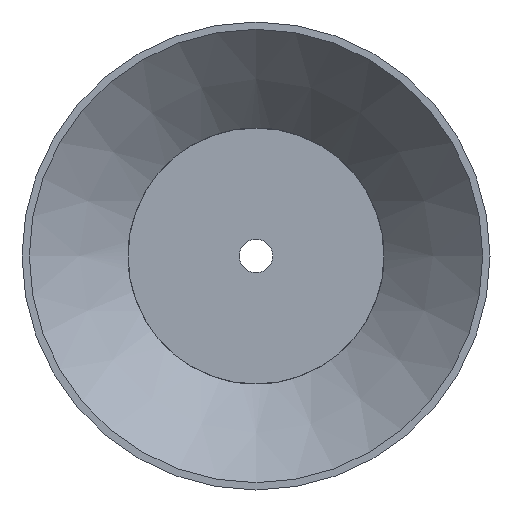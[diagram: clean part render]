
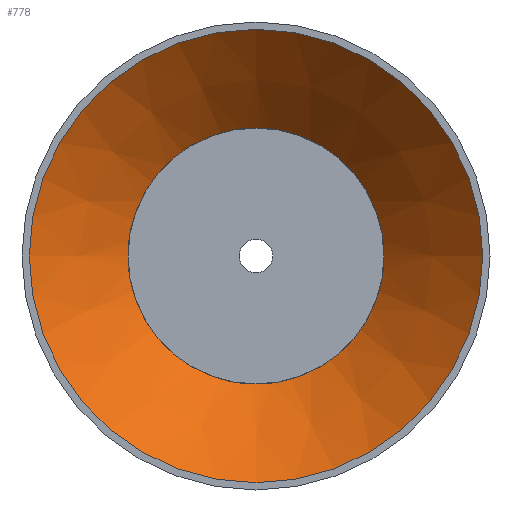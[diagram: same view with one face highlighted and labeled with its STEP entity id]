
A CAD part, front view. The second image highlights one B-rep face of the part: STEP entity #778.
In plain terms, the highlighted conical face has half-angle 44.201 degrees and reference radius 30.725 mm.
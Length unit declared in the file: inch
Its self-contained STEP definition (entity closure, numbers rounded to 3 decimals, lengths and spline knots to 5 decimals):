
#110=(
BOUNDED_CURVE()
B_SPLINE_CURVE(2,(#1062,#1063,#1064),.UNSPECIFIED.,.F.,.F.)
B_SPLINE_CURVE_WITH_KNOTS((3,3),(0.,0.02415),.UNSPECIFIED.)
CURVE()
GEOMETRIC_REPRESENTATION_ITEM()
RATIONAL_B_SPLINE_CURVE((1.,1.,1.))
REPRESENTATION_ITEM('')
);
#111=(
BOUNDED_CURVE()
B_SPLINE_CURVE(2,(#1066,#1067,#1068),.UNSPECIFIED.,.F.,.F.)
B_SPLINE_CURVE_WITH_KNOTS((3,3),(1.03572,1.05987),
 .UNSPECIFIED.)
CURVE()
GEOMETRIC_REPRESENTATION_ITEM()
RATIONAL_B_SPLINE_CURVE((1.,1.,1.))
REPRESENTATION_ITEM('')
);
#112=(
BOUNDED_CURVE()
B_SPLINE_CURVE(2,(#1071,#1072,#1073),.UNSPECIFIED.,.F.,.F.)
B_SPLINE_CURVE_WITH_KNOTS((3,3),(0.,0.02414),.UNSPECIFIED.)
CURVE()
GEOMETRIC_REPRESENTATION_ITEM()
RATIONAL_B_SPLINE_CURVE((1.,1.,1.))
REPRESENTATION_ITEM('')
);
#113=(
BOUNDED_CURVE()
B_SPLINE_CURVE(2,(#1075,#1076,#1077),.UNSPECIFIED.,.F.,.F.)
B_SPLINE_CURVE_WITH_KNOTS((3,3),(1.03572,1.05987),
 .UNSPECIFIED.)
CURVE()
GEOMETRIC_REPRESENTATION_ITEM()
RATIONAL_B_SPLINE_CURVE((1.,1.,1.))
REPRESENTATION_ITEM('')
);
#114=(
BOUNDED_CURVE()
B_SPLINE_CURVE(2,(#1080,#1081,#1082),.UNSPECIFIED.,.F.,.F.)
B_SPLINE_CURVE_WITH_KNOTS((3,3),(0.,0.02414),.UNSPECIFIED.)
CURVE()
GEOMETRIC_REPRESENTATION_ITEM()
RATIONAL_B_SPLINE_CURVE((1.,1.,1.))
REPRESENTATION_ITEM('')
);
#115=(
BOUNDED_CURVE()
B_SPLINE_CURVE(2,(#1084,#1085,#1086),.UNSPECIFIED.,.F.,.F.)
B_SPLINE_CURVE_WITH_KNOTS((3,3),(1.03578,1.05992),
 .UNSPECIFIED.)
CURVE()
GEOMETRIC_REPRESENTATION_ITEM()
RATIONAL_B_SPLINE_CURVE((1.,1.,1.))
REPRESENTATION_ITEM('')
);
#116=(
BOUNDED_CURVE()
B_SPLINE_CURVE(2,(#1090,#1091,#1092),.UNSPECIFIED.,.F.,.F.)
B_SPLINE_CURVE_WITH_KNOTS((3,3),(0.,0.02414),.UNSPECIFIED.)
CURVE()
GEOMETRIC_REPRESENTATION_ITEM()
RATIONAL_B_SPLINE_CURVE((1.,1.,1.))
REPRESENTATION_ITEM('')
);
#117=(
BOUNDED_CURVE()
B_SPLINE_CURVE(2,(#1096,#1097,#1098),.UNSPECIFIED.,.F.,.F.)
B_SPLINE_CURVE_WITH_KNOTS((3,3),(1.03571,1.05985),
 .UNSPECIFIED.)
CURVE()
GEOMETRIC_REPRESENTATION_ITEM()
RATIONAL_B_SPLINE_CURVE((1.,1.,1.))
REPRESENTATION_ITEM('')
);
#119=CONICAL_SURFACE('',#834,1.20963,0.771);
#124=FACE_OUTER_BOUND('',#160,.T.);
#160=EDGE_LOOP('',(#513,#514,#515,#516,#517,#518,#519,#520,#521,#522,#523,
#524,#525,#526,#527,#528,#529,#530,#531,#532,#533));
#197=CIRCLE('',#827,0.86927);
#199=CIRCLE('',#830,0.86927);
#200=CIRCLE('',#832,0.86927);
#202=CIRCLE('',#835,1.55);
#203=CIRCLE('',#836,0.875);
#204=CIRCLE('',#837,0.875);
#205=CIRCLE('',#838,0.875);
#206=CIRCLE('',#839,0.875);
#207=CIRCLE('',#840,0.86927);
#208=CIRCLE('',#841,0.875);
#209=CIRCLE('',#842,1.55);
#238=LINE('',#1059,#260);
#260=VECTOR('',#914,1.20963);
#277=VERTEX_POINT('',#1029);
#279=VERTEX_POINT('',#1033);
#281=VERTEX_POINT('',#1038);
#283=VERTEX_POINT('',#1042);
#284=VERTEX_POINT('',#1046);
#286=VERTEX_POINT('',#1049);
#288=VERTEX_POINT('',#1055);
#289=VERTEX_POINT('',#1056);
#290=VERTEX_POINT('',#1058);
#291=VERTEX_POINT('',#1060);
#292=VERTEX_POINT('',#1065);
#293=VERTEX_POINT('',#1069);
#294=VERTEX_POINT('',#1074);
#295=VERTEX_POINT('',#1078);
#296=VERTEX_POINT('',#1083);
#297=VERTEX_POINT('',#1087);
#298=VERTEX_POINT('',#1089);
#299=VERTEX_POINT('',#1093);
#300=VERTEX_POINT('',#1095);
#371=EDGE_CURVE('',#279,#277,#197,.T.);
#375=EDGE_CURVE('',#283,#281,#199,.T.);
#377=EDGE_CURVE('',#284,#286,#200,.T.);
#380=EDGE_CURVE('',#288,#289,#202,.T.);
#381=EDGE_CURVE('',#289,#290,#238,.T.);
#382=EDGE_CURVE('',#291,#290,#203,.T.);
#383=EDGE_CURVE('',#281,#291,#110,.T.);
#384=EDGE_CURVE('',#292,#283,#111,.T.);
#385=EDGE_CURVE('',#293,#292,#204,.T.);
#386=EDGE_CURVE('',#277,#293,#112,.T.);
#387=EDGE_CURVE('',#294,#279,#113,.T.);
#388=EDGE_CURVE('',#295,#294,#205,.T.);
#389=EDGE_CURVE('',#286,#295,#114,.T.);
#390=EDGE_CURVE('',#296,#284,#115,.T.);
#391=EDGE_CURVE('',#297,#296,#206,.T.);
#392=EDGE_CURVE('',#298,#297,#116,.T.);
#393=EDGE_CURVE('',#299,#298,#207,.T.);
#394=EDGE_CURVE('',#300,#299,#117,.T.);
#395=EDGE_CURVE('',#290,#300,#208,.T.);
#396=EDGE_CURVE('',#289,#288,#209,.T.);
#513=ORIENTED_EDGE('',*,*,#380,.T.);
#514=ORIENTED_EDGE('',*,*,#381,.T.);
#515=ORIENTED_EDGE('',*,*,#382,.F.);
#516=ORIENTED_EDGE('',*,*,#383,.F.);
#517=ORIENTED_EDGE('',*,*,#375,.F.);
#518=ORIENTED_EDGE('',*,*,#384,.F.);
#519=ORIENTED_EDGE('',*,*,#385,.F.);
#520=ORIENTED_EDGE('',*,*,#386,.F.);
#521=ORIENTED_EDGE('',*,*,#371,.F.);
#522=ORIENTED_EDGE('',*,*,#387,.F.);
#523=ORIENTED_EDGE('',*,*,#388,.F.);
#524=ORIENTED_EDGE('',*,*,#389,.F.);
#525=ORIENTED_EDGE('',*,*,#377,.F.);
#526=ORIENTED_EDGE('',*,*,#390,.F.);
#527=ORIENTED_EDGE('',*,*,#391,.F.);
#528=ORIENTED_EDGE('',*,*,#392,.F.);
#529=ORIENTED_EDGE('',*,*,#393,.F.);
#530=ORIENTED_EDGE('',*,*,#394,.F.);
#531=ORIENTED_EDGE('',*,*,#395,.F.);
#532=ORIENTED_EDGE('',*,*,#381,.F.);
#533=ORIENTED_EDGE('',*,*,#396,.T.);
#778=ADVANCED_FACE('',(#124),#119,.F.);
#827=AXIS2_PLACEMENT_3D('',#1035,#892,#893);
#830=AXIS2_PLACEMENT_3D('',#1044,#900,#901);
#832=AXIS2_PLACEMENT_3D('',#1050,#905,#906);
#834=AXIS2_PLACEMENT_3D('',#1054,#910,#911);
#835=AXIS2_PLACEMENT_3D('',#1057,#912,#913);
#836=AXIS2_PLACEMENT_3D('',#1061,#915,#916);
#837=AXIS2_PLACEMENT_3D('',#1070,#917,#918);
#838=AXIS2_PLACEMENT_3D('',#1079,#919,#920);
#839=AXIS2_PLACEMENT_3D('',#1088,#921,#922);
#840=AXIS2_PLACEMENT_3D('',#1094,#923,#924);
#841=AXIS2_PLACEMENT_3D('',#1099,#925,#926);
#842=AXIS2_PLACEMENT_3D('',#1100,#927,#928);
#892=DIRECTION('center_axis',(0.,-1.,0.));
#893=DIRECTION('ref_axis',(1.,0.,0.));
#900=DIRECTION('center_axis',(0.,-1.,0.));
#901=DIRECTION('ref_axis',(1.,0.,0.));
#905=DIRECTION('center_axis',(0.,-1.,0.));
#906=DIRECTION('ref_axis',(1.,0.,0.));
#910=DIRECTION('center_axis',(0.,-1.,0.));
#911=DIRECTION('ref_axis',(1.,0.,0.));
#912=DIRECTION('center_axis',(0.,-1.,0.));
#913=DIRECTION('ref_axis',(1.,0.,0.));
#914=DIRECTION('',(0.697,0.717,0.));
#915=DIRECTION('center_axis',(0.,-1.,0.));
#916=DIRECTION('ref_axis',(1.,0.,0.));
#917=DIRECTION('center_axis',(0.,-1.,0.));
#918=DIRECTION('ref_axis',(1.,0.,0.));
#919=DIRECTION('center_axis',(0.,-1.,0.));
#920=DIRECTION('ref_axis',(1.,0.,0.));
#921=DIRECTION('center_axis',(0.,-1.,0.));
#922=DIRECTION('ref_axis',(1.,0.,0.));
#923=DIRECTION('center_axis',(0.,-1.,0.));
#924=DIRECTION('ref_axis',(1.,0.,0.));
#925=DIRECTION('center_axis',(0.,-1.,0.));
#926=DIRECTION('ref_axis',(1.,0.,0.));
#927=DIRECTION('center_axis',(0.,-1.,0.));
#928=DIRECTION('ref_axis',(1.,0.,0.));
#1029=CARTESIAN_POINT('',(0.10004,0.7,0.86349));
#1033=CARTESIAN_POINT('',(0.8635,0.7,0.1));
#1035=CARTESIAN_POINT('Origin',(0.,0.7,0.));
#1038=CARTESIAN_POINT('',(-0.8635,0.7,0.09997));
#1042=CARTESIAN_POINT('',(-0.1,0.7,0.8635));
#1044=CARTESIAN_POINT('Origin',(0.,0.7,0.));
#1046=CARTESIAN_POINT('',(0.09992,0.7,-0.8635));
#1049=CARTESIAN_POINT('',(0.86348,0.7,-0.10016));
#1050=CARTESIAN_POINT('Origin',(0.,0.7,0.));
#1054=CARTESIAN_POINT('Origin',(0.,0.35,0.));
#1055=CARTESIAN_POINT('',(1.55,0.,0.));
#1056=CARTESIAN_POINT('',(-1.55,0.,0.));
#1057=CARTESIAN_POINT('Origin',(0.,0.,0.));
#1058=CARTESIAN_POINT('',(-0.875,0.6941,0.));
#1059=CARTESIAN_POINT('',(-1.20963,0.35,0.));
#1060=CARTESIAN_POINT('',(-0.86927,0.6941,0.09997));
#1061=CARTESIAN_POINT('Origin',(0.,0.6941,0.));
#1062=CARTESIAN_POINT('Ctrl Pts',(-0.8635,0.7,0.09997));
#1063=CARTESIAN_POINT('Ctrl Pts',(-0.86638,0.69706,
0.09997));
#1064=CARTESIAN_POINT('Ctrl Pts',(-0.86927,0.6941,
0.09997));
#1065=CARTESIAN_POINT('',(-0.1,0.6941,0.86927));
#1066=CARTESIAN_POINT('Ctrl Pts',(-0.1,0.6941,0.86927));
#1067=CARTESIAN_POINT('Ctrl Pts',(-0.1,0.69706,0.86637));
#1068=CARTESIAN_POINT('Ctrl Pts',(-0.1,0.7,0.8635));
#1069=CARTESIAN_POINT('',(0.10004,0.6941,0.86926));
#1070=CARTESIAN_POINT('Origin',(0.,0.6941,0.));
#1071=CARTESIAN_POINT('Ctrl Pts',(0.10004,0.7,0.86349));
#1072=CARTESIAN_POINT('Ctrl Pts',(0.10004,0.69706,0.86637));
#1073=CARTESIAN_POINT('Ctrl Pts',(0.10004,0.6941,0.86926));
#1074=CARTESIAN_POINT('',(0.86927,0.6941,0.1));
#1075=CARTESIAN_POINT('Ctrl Pts',(0.86927,0.6941,0.1));
#1076=CARTESIAN_POINT('Ctrl Pts',(0.86637,0.69706,0.1));
#1077=CARTESIAN_POINT('Ctrl Pts',(0.8635,0.7,0.1));
#1078=CARTESIAN_POINT('',(0.86925,0.6941,-0.10017));
#1079=CARTESIAN_POINT('Origin',(0.,0.6941,0.));
#1080=CARTESIAN_POINT('Ctrl Pts',(0.86348,0.7,-0.10016));
#1081=CARTESIAN_POINT('Ctrl Pts',(0.86635,0.69706,-0.10016));
#1082=CARTESIAN_POINT('Ctrl Pts',(0.86925,0.6941,-0.10017));
#1083=CARTESIAN_POINT('',(0.09992,0.6941,-0.86928));
#1084=CARTESIAN_POINT('Ctrl Pts',(0.09992,0.6941,
-0.86928));
#1085=CARTESIAN_POINT('Ctrl Pts',(0.09992,0.69706,
-0.86638));
#1086=CARTESIAN_POINT('Ctrl Pts',(0.09992,0.7,
-0.8635));
#1087=CARTESIAN_POINT('',(-0.10001,0.6941,-0.86927));
#1088=CARTESIAN_POINT('Origin',(0.,0.6941,0.));
#1089=CARTESIAN_POINT('',(-0.10001,0.7,-0.86349));
#1090=CARTESIAN_POINT('Ctrl Pts',(-0.10001,0.7,
-0.86349));
#1091=CARTESIAN_POINT('Ctrl Pts',(-0.10001,0.69706,
-0.86637));
#1092=CARTESIAN_POINT('Ctrl Pts',(-0.10001,0.6941,
-0.86927));
#1093=CARTESIAN_POINT('',(-0.86349,0.7,-0.10002));
#1094=CARTESIAN_POINT('Origin',(0.,0.7,0.));
#1095=CARTESIAN_POINT('',(-0.86926,0.6941,-0.10002));
#1096=CARTESIAN_POINT('Ctrl Pts',(-0.86926,0.6941,
-0.10002));
#1097=CARTESIAN_POINT('Ctrl Pts',(-0.86637,0.69706,
-0.10002));
#1098=CARTESIAN_POINT('Ctrl Pts',(-0.86349,0.7,
-0.10002));
#1099=CARTESIAN_POINT('Origin',(0.,0.6941,0.));
#1100=CARTESIAN_POINT('Origin',(0.,0.,0.));
